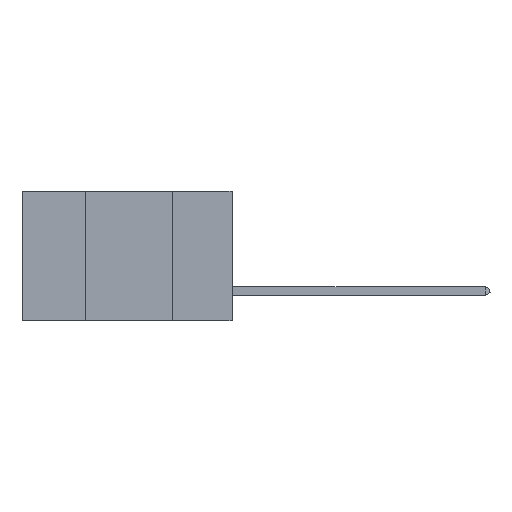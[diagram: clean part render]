
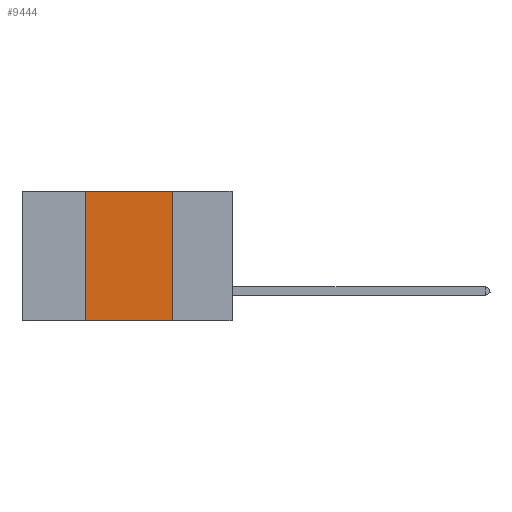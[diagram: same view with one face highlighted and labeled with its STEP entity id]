
A CAD part, left-side view. The second image highlights one B-rep face of the part: STEP entity #9444.
In plain terms, the highlighted planar face has unit normal (-1, 0, 0).
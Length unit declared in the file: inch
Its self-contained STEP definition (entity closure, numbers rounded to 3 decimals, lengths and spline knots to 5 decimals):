
#810 = ORIENTED_EDGE ( 'NONE', *, *, #839, .F. ) ;
#839 = EDGE_CURVE ( 'NONE', #27752, #4954, #42134, .T. ) ;
#2507 = CARTESIAN_POINT ( 'NONE',  ( 0., 0.6, -0.37 ) ) ;
#4954 = VERTEX_POINT ( 'NONE', #41970 ) ;
#7245 = DIRECTION ( 'NONE',  ( 0., 0., -1. ) ) ;
#7917 = ORIENTED_EDGE ( 'NONE', *, *, #20069, .F. ) ;
#8333 = VERTEX_POINT ( 'NONE', #20358 ) ;
#9444 = ADVANCED_FACE ( 'NONE', ( #35661 ), #24596, .F. ) ;
#11959 = LINE ( 'NONE', #30183, #35260 ) ;
#13453 = LINE ( 'NONE', #22641, #37355 ) ;
#13872 = DIRECTION ( 'NONE',  ( 0., -1., 0. ) ) ;
#16940 = DIRECTION ( 'NONE',  ( 0., 0., -1. ) ) ;
#20069 = EDGE_CURVE ( 'NONE', #4954, #8333, #13453, .T. ) ;
#20358 = CARTESIAN_POINT ( 'NONE',  ( 0., 0.17, 0. ) ) ;
#21215 = CARTESIAN_POINT ( 'NONE',  ( 0., 0.17, -0.37 ) ) ;
#21932 = AXIS2_PLACEMENT_3D ( 'NONE', #28644, #28134, #16940 ) ;
#22546 = EDGE_CURVE ( 'NONE', #8333, #43432, #11959, .T. ) ;
#22641 = CARTESIAN_POINT ( 'NONE',  ( 0., 0.6, 0. ) ) ;
#22798 = DIRECTION ( 'NONE',  ( 0., -1., 0. ) ) ;
#24596 = PLANE ( 'NONE',  #21932 ) ;
#27752 = VERTEX_POINT ( 'NONE', #42810 ) ;
#28134 = DIRECTION ( 'NONE',  ( 1., 0., 0. ) ) ;
#28644 = CARTESIAN_POINT ( 'NONE',  ( 0., 0.6, 0. ) ) ;
#29956 = EDGE_CURVE ( 'NONE', #27752, #43432, #48416, .T. ) ;
#30183 = CARTESIAN_POINT ( 'NONE',  ( 0., 0.17, 0. ) ) ;
#33975 = CARTESIAN_POINT ( 'NONE',  ( 0., 0.42, 0. ) ) ;
#35260 = VECTOR ( 'NONE', #7245, 39.37008 ) ;
#35316 = EDGE_LOOP ( 'NONE', ( #35446, #7917, #810, #37797 ) ) ;
#35446 = ORIENTED_EDGE ( 'NONE', *, *, #22546, .F. ) ;
#35661 = FACE_OUTER_BOUND ( 'NONE', #35316, .T. ) ;
#36737 = VECTOR ( 'NONE', #38102, 39.37008 ) ;
#37355 = VECTOR ( 'NONE', #22798, 39.37008 ) ;
#37797 = ORIENTED_EDGE ( 'NONE', *, *, #29956, .T. ) ;
#38102 = DIRECTION ( 'NONE',  ( 0., 0., 1. ) ) ;
#38240 = VECTOR ( 'NONE', #13872, 39.37008 ) ;
#41970 = CARTESIAN_POINT ( 'NONE',  ( 0., 0.42, 0. ) ) ;
#42134 = LINE ( 'NONE', #33975, #36737 ) ;
#42810 = CARTESIAN_POINT ( 'NONE',  ( 0., 0.42, -0.37 ) ) ;
#43432 = VERTEX_POINT ( 'NONE', #21215 ) ;
#48416 = LINE ( 'NONE', #2507, #38240 ) ;
